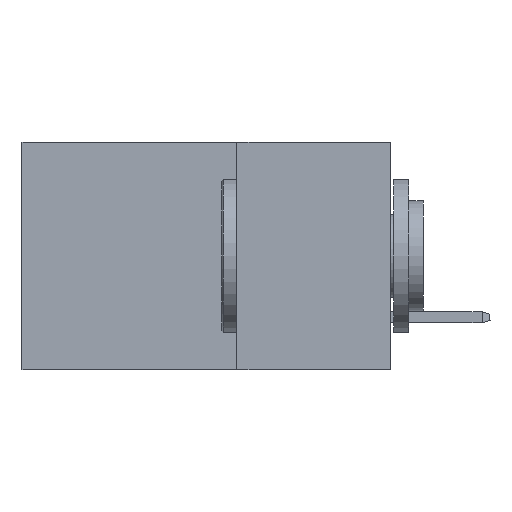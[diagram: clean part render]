
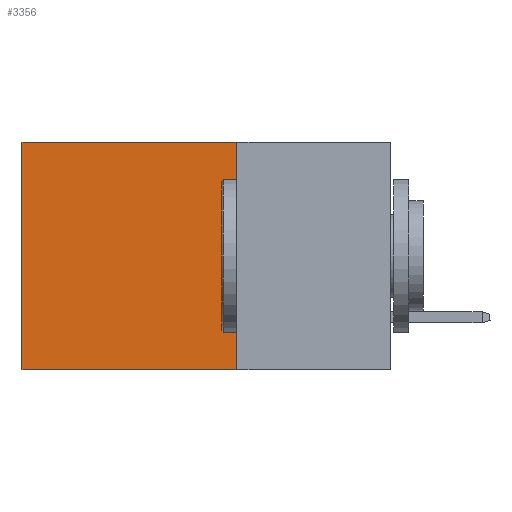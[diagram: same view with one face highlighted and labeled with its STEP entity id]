
A CAD part, left-side view. The second image highlights one B-rep face of the part: STEP entity #3356.
In plain terms, the highlighted planar face has unit normal (-1, 0, 0).
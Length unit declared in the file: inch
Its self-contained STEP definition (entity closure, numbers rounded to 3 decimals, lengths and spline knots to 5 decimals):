
#128 = CARTESIAN_POINT ( 'NONE',  ( 0.2875, 0.25, -0.37 ) ) ;
#148 = VERTEX_POINT ( 'NONE', #20538 ) ;
#283 = LINE ( 'NONE', #128, #18899 ) ;
#315 = VERTEX_POINT ( 'NONE', #2040 ) ;
#1444 = LINE ( 'NONE', #24781, #24881 ) ;
#1674 = CARTESIAN_POINT ( 'NONE',  ( 0.2875, 0.25, -0.37 ) ) ;
#2040 = CARTESIAN_POINT ( 'NONE',  ( 0.2875, 0.25, 0. ) ) ;
#3356 = ADVANCED_FACE ( 'NONE', ( #13601 ), #3812, .F. ) ;
#3812 = PLANE ( 'NONE',  #16081 ) ;
#4323 = LINE ( 'NONE', #6110, #20785 ) ;
#5452 = LINE ( 'NONE', #18068, #8884 ) ;
#5723 = DIRECTION ( 'NONE',  ( 1., 0., 0. ) ) ;
#6110 = CARTESIAN_POINT ( 'NONE',  ( 0.2875, 0.25, 0. ) ) ;
#7741 = CARTESIAN_POINT ( 'NONE',  ( 0.2875, 0.6, 0. ) ) ;
#8447 = DIRECTION ( 'NONE',  ( 0., 1., 0. ) ) ;
#8884 = VECTOR ( 'NONE', #15947, 39.37008 ) ;
#10973 = ORIENTED_EDGE ( 'NONE', *, *, #23724, .T. ) ;
#11802 = DIRECTION ( 'NONE',  ( 0., 0., -1. ) ) ;
#13090 = VERTEX_POINT ( 'NONE', #1674 ) ;
#13601 = FACE_OUTER_BOUND ( 'NONE', #21761, .T. ) ;
#15861 = ORIENTED_EDGE ( 'NONE', *, *, #22962, .F. ) ;
#15947 = DIRECTION ( 'NONE',  ( 0., 0., -1. ) ) ;
#16081 = AXIS2_PLACEMENT_3D ( 'NONE', #23538, #5723, #11802 ) ;
#17215 = EDGE_CURVE ( 'NONE', #315, #25498, #4323, .T. ) ;
#18068 = CARTESIAN_POINT ( 'NONE',  ( 0.2875, 0.25, 0. ) ) ;
#18899 = VECTOR ( 'NONE', #21762, 39.37008 ) ;
#20538 = CARTESIAN_POINT ( 'NONE',  ( 0.2875, 0.6, -0.37 ) ) ;
#20633 = EDGE_CURVE ( 'NONE', #13090, #148, #283, .T. ) ;
#20785 = VECTOR ( 'NONE', #8447, 39.37008 ) ;
#21693 = ORIENTED_EDGE ( 'NONE', *, *, #20633, .F. ) ;
#21761 = EDGE_LOOP ( 'NONE', ( #10973, #21693, #15861, #25127 ) ) ;
#21762 = DIRECTION ( 'NONE',  ( 0., 1., 0. ) ) ;
#22962 = EDGE_CURVE ( 'NONE', #315, #13090, #5452, .T. ) ;
#23538 = CARTESIAN_POINT ( 'NONE',  ( 0.2875, 0.25, 0. ) ) ;
#23724 = EDGE_CURVE ( 'NONE', #25498, #148, #1444, .T. ) ;
#24705 = DIRECTION ( 'NONE',  ( 0., 0., -1. ) ) ;
#24781 = CARTESIAN_POINT ( 'NONE',  ( 0.2875, 0.6, 0. ) ) ;
#24881 = VECTOR ( 'NONE', #24705, 39.37008 ) ;
#25127 = ORIENTED_EDGE ( 'NONE', *, *, #17215, .T. ) ;
#25498 = VERTEX_POINT ( 'NONE', #7741 ) ;
